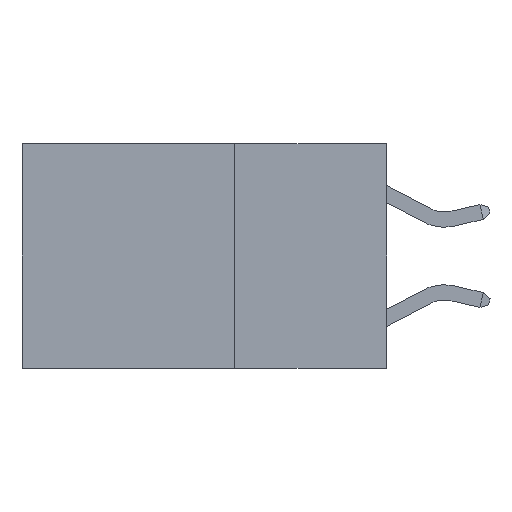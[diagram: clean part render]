
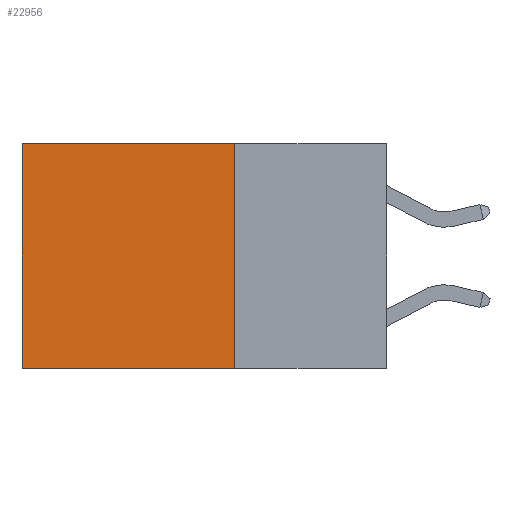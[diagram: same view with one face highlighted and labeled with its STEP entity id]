
A CAD part, left-side view. The second image highlights one B-rep face of the part: STEP entity #22956.
In plain terms, the highlighted planar face has unit normal (-1, 0, 0).
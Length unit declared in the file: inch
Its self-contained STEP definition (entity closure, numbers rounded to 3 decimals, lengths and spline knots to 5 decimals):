
#1187 = LINE ( 'NONE', #28885, #6717 ) ;
#1419 = CARTESIAN_POINT ( 'NONE',  ( 0.2625, 0.25, 0. ) ) ;
#2181 = CARTESIAN_POINT ( 'NONE',  ( 0.2625, 0.25, 0. ) ) ;
#3541 = CARTESIAN_POINT ( 'NONE',  ( 0.2625, 0.6, -0.37 ) ) ;
#4402 = VECTOR ( 'NONE', #10965, 39.37008 ) ;
#5805 = VERTEX_POINT ( 'NONE', #6248 ) ;
#6248 = CARTESIAN_POINT ( 'NONE',  ( 0.2625, 0.25, -0.37 ) ) ;
#6312 = CARTESIAN_POINT ( 'NONE',  ( 0.2625, 0.6, 0. ) ) ;
#6717 = VECTOR ( 'NONE', #15034, 39.37008 ) ;
#7597 = EDGE_CURVE ( 'NONE', #5805, #23820, #1187, .T. ) ;
#7836 = ORIENTED_EDGE ( 'NONE', *, *, #9097, .T. ) ;
#8916 = LINE ( 'NONE', #1419, #26778 ) ;
#9097 = EDGE_CURVE ( 'NONE', #25336, #23820, #22362, .T. ) ;
#9976 = PLANE ( 'NONE',  #24583 ) ;
#10375 = ORIENTED_EDGE ( 'NONE', *, *, #7597, .F. ) ;
#10965 = DIRECTION ( 'NONE',  ( 0., 0., -1. ) ) ;
#11601 = DIRECTION ( 'NONE',  ( 0., 1., 0. ) ) ;
#12363 = DIRECTION ( 'NONE',  ( 0., 0., -1. ) ) ;
#13817 = VECTOR ( 'NONE', #11601, 39.37008 ) ;
#14511 = FACE_OUTER_BOUND ( 'NONE', #20253, .T. ) ;
#15034 = DIRECTION ( 'NONE',  ( 0., 1., 0. ) ) ;
#15224 = EDGE_CURVE ( 'NONE', #19241, #25336, #19953, .T. ) ;
#15563 = DIRECTION ( 'NONE',  ( 0., 0., -1. ) ) ;
#16594 = EDGE_CURVE ( 'NONE', #19241, #5805, #8916, .T. ) ;
#19241 = VERTEX_POINT ( 'NONE', #2181 ) ;
#19256 = CARTESIAN_POINT ( 'NONE',  ( 0.2625, 0.25, 0. ) ) ;
#19953 = LINE ( 'NONE', #27728, #13817 ) ;
#20253 = EDGE_LOOP ( 'NONE', ( #7836, #10375, #20302, #24287 ) ) ;
#20302 = ORIENTED_EDGE ( 'NONE', *, *, #16594, .F. ) ;
#22362 = LINE ( 'NONE', #6312, #4402 ) ;
#22956 = ADVANCED_FACE ( 'NONE', ( #14511 ), #9976, .F. ) ;
#23820 = VERTEX_POINT ( 'NONE', #3541 ) ;
#24287 = ORIENTED_EDGE ( 'NONE', *, *, #15224, .T. ) ;
#24583 = AXIS2_PLACEMENT_3D ( 'NONE', #19256, #26229, #12363 ) ;
#25336 = VERTEX_POINT ( 'NONE', #30143 ) ;
#26229 = DIRECTION ( 'NONE',  ( 1., 0., 0. ) ) ;
#26778 = VECTOR ( 'NONE', #15563, 39.37008 ) ;
#27728 = CARTESIAN_POINT ( 'NONE',  ( 0.2625, 0.25, 0. ) ) ;
#28885 = CARTESIAN_POINT ( 'NONE',  ( 0.2625, 0.25, -0.37 ) ) ;
#30143 = CARTESIAN_POINT ( 'NONE',  ( 0.2625, 0.6, 0. ) ) ;
